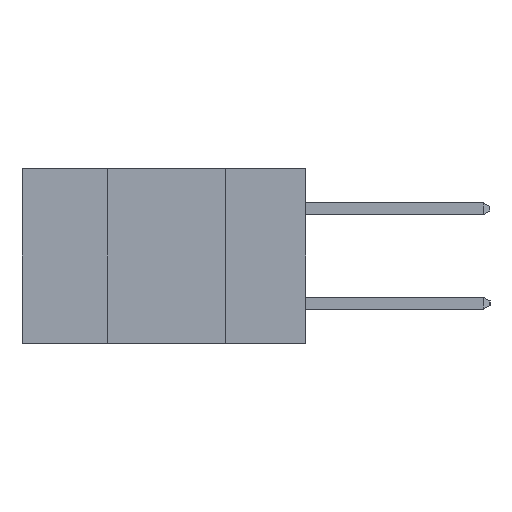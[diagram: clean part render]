
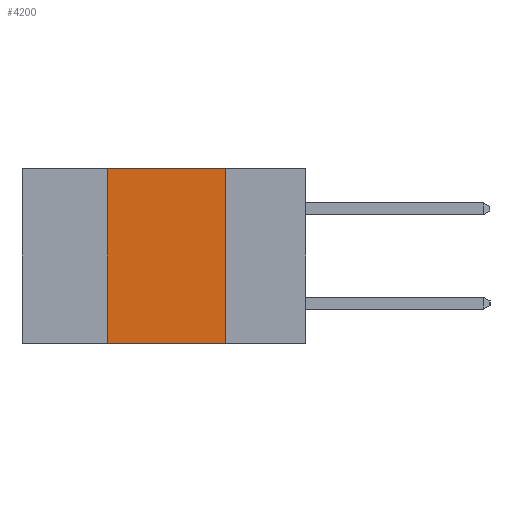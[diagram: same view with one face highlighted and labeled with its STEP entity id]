
A CAD part, left-side view. The second image highlights one B-rep face of the part: STEP entity #4200.
In plain terms, the highlighted planar face has unit normal (-1, 0, 0).
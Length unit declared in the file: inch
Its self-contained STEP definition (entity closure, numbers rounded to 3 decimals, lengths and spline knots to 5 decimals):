
#372 = CARTESIAN_POINT ( 'NONE',  ( 0., 0.17, -0.37 ) ) ;
#1620 = DIRECTION ( 'NONE',  ( 0., -1., 0. ) ) ;
#1688 = CARTESIAN_POINT ( 'NONE',  ( 0., 0.6, -0.37 ) ) ;
#1871 = VECTOR ( 'NONE', #12907, 39.37008 ) ;
#2248 = VERTEX_POINT ( 'NONE', #4871 ) ;
#2527 = ORIENTED_EDGE ( 'NONE', *, *, #16483, .F. ) ;
#2686 = EDGE_CURVE ( 'NONE', #2248, #11576, #2716, .T. ) ;
#2716 = LINE ( 'NONE', #12603, #1871 ) ;
#4009 = LINE ( 'NONE', #6729, #10717 ) ;
#4200 = ADVANCED_FACE ( 'NONE', ( #11669 ), #11465, .F. ) ;
#4871 = CARTESIAN_POINT ( 'NONE',  ( 0., 0.42, 0. ) ) ;
#5380 = LINE ( 'NONE', #1688, #15338 ) ;
#6341 = LINE ( 'NONE', #8194, #16185 ) ;
#6729 = CARTESIAN_POINT ( 'NONE',  ( 0., 0.42, -0.37 ) ) ;
#6846 = DIRECTION ( 'NONE',  ( 0., 0., -1. ) ) ;
#8194 = CARTESIAN_POINT ( 'NONE',  ( 0., 0.17, -0.37 ) ) ;
#8798 = VERTEX_POINT ( 'NONE', #13881 ) ;
#8855 = EDGE_LOOP ( 'NONE', ( #13093, #11118, #2527, #11766 ) ) ;
#9305 = EDGE_CURVE ( 'NONE', #8798, #16014, #5380, .T. ) ;
#10717 = VECTOR ( 'NONE', #14516, 39.37008 ) ;
#11118 = ORIENTED_EDGE ( 'NONE', *, *, #2686, .F. ) ;
#11162 = DIRECTION ( 'NONE',  ( 0., 0., -1. ) ) ;
#11228 = DIRECTION ( 'NONE',  ( 1., 0., 0. ) ) ;
#11279 = CARTESIAN_POINT ( 'NONE',  ( 0., 0.6, 0. ) ) ;
#11412 = AXIS2_PLACEMENT_3D ( 'NONE', #11279, #11228, #11162 ) ;
#11465 = PLANE ( 'NONE',  #11412 ) ;
#11576 = VERTEX_POINT ( 'NONE', #14807 ) ;
#11669 = FACE_OUTER_BOUND ( 'NONE', #8855, .T. ) ;
#11766 = ORIENTED_EDGE ( 'NONE', *, *, #9305, .T. ) ;
#12603 = CARTESIAN_POINT ( 'NONE',  ( 0., 0.6, 0. ) ) ;
#12907 = DIRECTION ( 'NONE',  ( 0., -1., 0. ) ) ;
#13093 = ORIENTED_EDGE ( 'NONE', *, *, #16536, .F. ) ;
#13881 = CARTESIAN_POINT ( 'NONE',  ( 0., 0.42, -0.37 ) ) ;
#14516 = DIRECTION ( 'NONE',  ( 0., 0., 1. ) ) ;
#14807 = CARTESIAN_POINT ( 'NONE',  ( 0., 0.17, 0. ) ) ;
#15338 = VECTOR ( 'NONE', #1620, 39.37008 ) ;
#16014 = VERTEX_POINT ( 'NONE', #372 ) ;
#16185 = VECTOR ( 'NONE', #6846, 39.37008 ) ;
#16483 = EDGE_CURVE ( 'NONE', #8798, #2248, #4009, .T. ) ;
#16536 = EDGE_CURVE ( 'NONE', #11576, #16014, #6341, .T. ) ;
